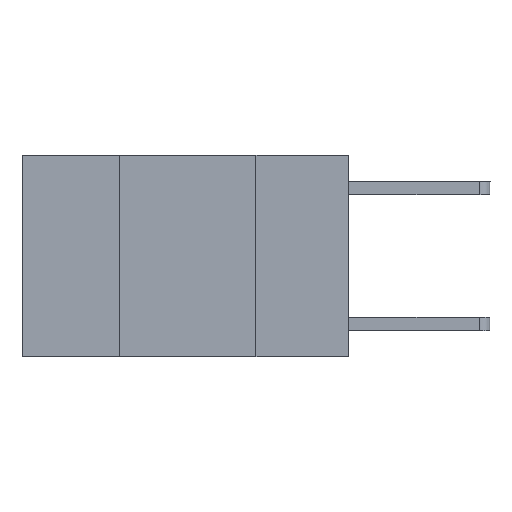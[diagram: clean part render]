
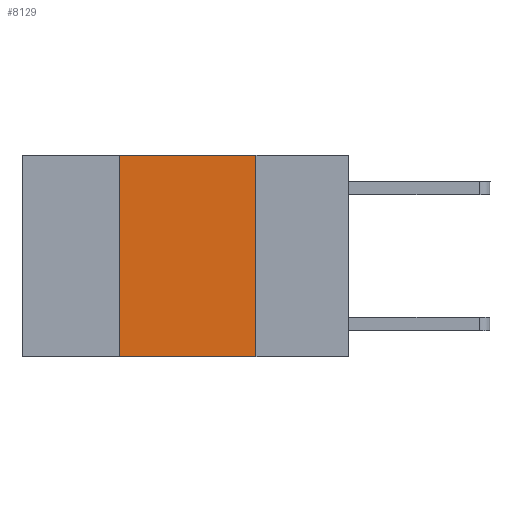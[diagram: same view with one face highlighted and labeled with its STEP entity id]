
A CAD part, left-side view. The second image highlights one B-rep face of the part: STEP entity #8129.
In plain terms, the highlighted planar face has unit normal (-1, 0, 0).
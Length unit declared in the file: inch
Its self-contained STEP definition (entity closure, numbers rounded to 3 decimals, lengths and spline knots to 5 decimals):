
#54 = VERTEX_POINT ( 'NONE', #7105 ) ;
#296 = VECTOR ( 'NONE', #3676, 39.37008 ) ;
#671 = DIRECTION ( 'NONE',  ( 1., 0., 0. ) ) ;
#884 = CARTESIAN_POINT ( 'NONE',  ( 0., 0.42, -0.37 ) ) ;
#1064 = EDGE_CURVE ( 'NONE', #7822, #5255, #2248, .T. ) ;
#1432 = FACE_OUTER_BOUND ( 'NONE', #8558, .T. ) ;
#1562 = EDGE_CURVE ( 'NONE', #2683, #54, #7900, .T. ) ;
#2248 = LINE ( 'NONE', #4959, #4650 ) ;
#2366 = CARTESIAN_POINT ( 'NONE',  ( 0., 0.17, -0.37 ) ) ;
#2683 = VERTEX_POINT ( 'NONE', #3599 ) ;
#2693 = EDGE_CURVE ( 'NONE', #7822, #2683, #4951, .T. ) ;
#3010 = AXIS2_PLACEMENT_3D ( 'NONE', #6856, #671, #6114 ) ;
#3138 = VECTOR ( 'NONE', #5376, 39.37008 ) ;
#3439 = VECTOR ( 'NONE', #4741, 39.37008 ) ;
#3533 = ORIENTED_EDGE ( 'NONE', *, *, #1562, .F. ) ;
#3599 = CARTESIAN_POINT ( 'NONE',  ( 0., 0.42, 0. ) ) ;
#3676 = DIRECTION ( 'NONE',  ( 0., 0., 1. ) ) ;
#4243 = PLANE ( 'NONE',  #3010 ) ;
#4650 = VECTOR ( 'NONE', #5012, 39.37008 ) ;
#4741 = DIRECTION ( 'NONE',  ( 0., 0., -1. ) ) ;
#4786 = LINE ( 'NONE', #7436, #3439 ) ;
#4951 = LINE ( 'NONE', #8379, #296 ) ;
#4959 = CARTESIAN_POINT ( 'NONE',  ( 0., 0.6, -0.37 ) ) ;
#4996 = ORIENTED_EDGE ( 'NONE', *, *, #6711, .F. ) ;
#5012 = DIRECTION ( 'NONE',  ( 0., -1., 0. ) ) ;
#5255 = VERTEX_POINT ( 'NONE', #2366 ) ;
#5376 = DIRECTION ( 'NONE',  ( 0., -1., 0. ) ) ;
#5659 = ORIENTED_EDGE ( 'NONE', *, *, #1064, .T. ) ;
#6114 = DIRECTION ( 'NONE',  ( 0., 0., -1. ) ) ;
#6711 = EDGE_CURVE ( 'NONE', #54, #5255, #4786, .T. ) ;
#6856 = CARTESIAN_POINT ( 'NONE',  ( 0., 0.6, 0. ) ) ;
#6975 = ORIENTED_EDGE ( 'NONE', *, *, #2693, .F. ) ;
#7105 = CARTESIAN_POINT ( 'NONE',  ( 0., 0.17, 0. ) ) ;
#7436 = CARTESIAN_POINT ( 'NONE',  ( 0., 0.17, 0. ) ) ;
#7822 = VERTEX_POINT ( 'NONE', #884 ) ;
#7900 = LINE ( 'NONE', #8635, #3138 ) ;
#8129 = ADVANCED_FACE ( 'NONE', ( #1432 ), #4243, .F. ) ;
#8379 = CARTESIAN_POINT ( 'NONE',  ( 0., 0.42, 0. ) ) ;
#8558 = EDGE_LOOP ( 'NONE', ( #4996, #3533, #6975, #5659 ) ) ;
#8635 = CARTESIAN_POINT ( 'NONE',  ( 0., 0.6, 0. ) ) ;
